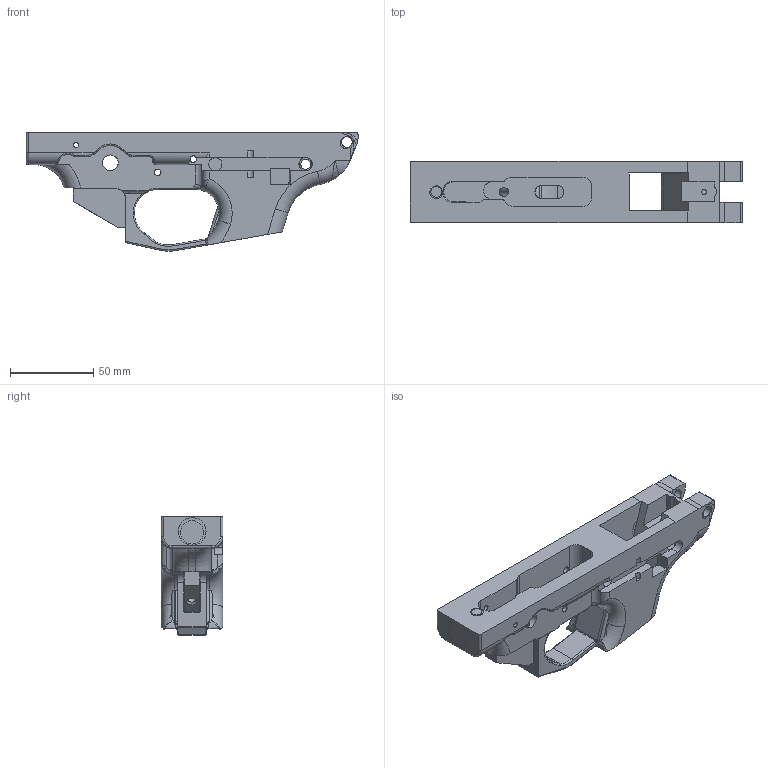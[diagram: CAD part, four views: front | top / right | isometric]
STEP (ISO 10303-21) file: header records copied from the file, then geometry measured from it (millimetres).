
FILE_DESCRIPTION(('FreeCAD Model'),'2;1');
FILE_NAME('ap9 gluty lower 2020.step','2020-04-04T17:47:18',('Author'),(''), 'Open CASCADE STEP processor 6.8','FreeCAD','Unknown');
FILE_SCHEMA(('AUTOMOTIVE_DESIGN_CC2 { 1 2 10303 214 -1 1 5 4 }'));
Products named in the file (1): Pocket034
Bounding box: 199.6 x 37.13 x 71.26 mm (x, y, z)
Volume: 160066 mm3; surface area: 51527.6 mm2
Topology: 1 solids, 2 shells, 425 faces, 1213 edges, 768 vertices
Faces by surface type: plane 203, cylinder 136, bspline 41, torus 40, cone 3, sphere 2
Full cylindrical faces by diameter (mm): 3 x1, 3.175 x3, 3.969 x4, 5.105 x1, 6 x1, 6.4 x2, 8 x1, 9.525 x2, 16.2 x1
Entity records: 74087 total; most frequent: CARTESIAN_POINT 53257, DIRECTION 3045, ORIENTED_EDGE 2392, PCURVE 2392, DEFINITIONAL_REPRESENTATION 2392, B_SPLINE_CURVE_WITH_KNOTS 1472, LINE 1462, VECTOR 1462
